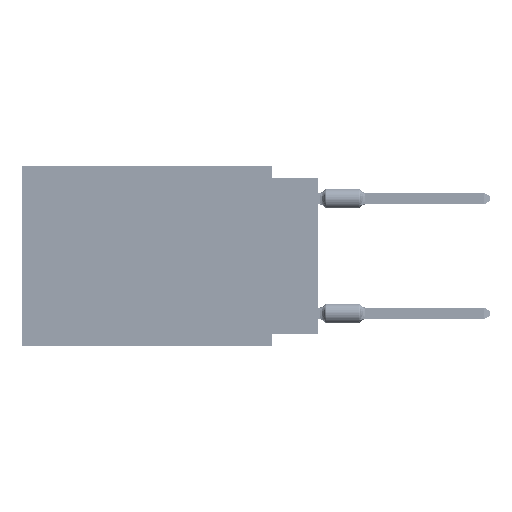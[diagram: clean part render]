
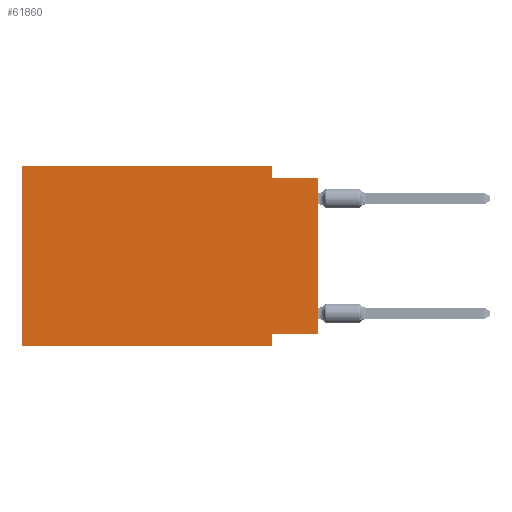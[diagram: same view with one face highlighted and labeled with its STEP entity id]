
A CAD part, left-side view. The second image highlights one B-rep face of the part: STEP entity #61860.
In plain terms, the highlighted planar face has unit normal (-1, 0, 0).
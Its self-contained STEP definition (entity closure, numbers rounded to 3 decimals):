
#1295 = VECTOR ( 'NONE', #41503, 1000. ) ;
#2583 = EDGE_CURVE ( 'NONE', #37512, #4246, #33294, .T. ) ;
#3146 = VERTEX_POINT ( 'NONE', #15341 ) ;
#3644 = ORIENTED_EDGE ( 'NONE', *, *, #2583, .T. ) ;
#4246 = VERTEX_POINT ( 'NONE', #16234 ) ;
#6691 = CARTESIAN_POINT ( 'NONE',  ( 0., 2.54, -0.635 ) ) ;
#6710 = LINE ( 'NONE', #60498, #7490 ) ;
#6810 = VERTEX_POINT ( 'NONE', #16343 ) ;
#7490 = VECTOR ( 'NONE', #61202, 1000. ) ;
#10549 = ORIENTED_EDGE ( 'NONE', *, *, #47215, .F. ) ;
#11896 = DIRECTION ( 'NONE',  ( 0., -1., 0. ) ) ;
#12000 = LINE ( 'NONE', #35159, #28196 ) ;
#12477 = EDGE_LOOP ( 'NONE', ( #29565, #55095, #37038, #61664, #54907, #3644, #34938, #10549 ) ) ;
#14765 = LINE ( 'NONE', #30801, #1295 ) ;
#14795 = VECTOR ( 'NONE', #61112, 1000. ) ;
#15341 = CARTESIAN_POINT ( 'NONE',  ( 0., 2.54, 0. ) ) ;
#16234 = CARTESIAN_POINT ( 'NONE',  ( 0., 2.54, -9.906 ) ) ;
#16343 = CARTESIAN_POINT ( 'NONE',  ( 0., 0., -9.271 ) ) ;
#18685 = CARTESIAN_POINT ( 'NONE',  ( 0., 0., 0. ) ) ;
#18696 = EDGE_CURVE ( 'NONE', #56143, #4246, #24344, .T. ) ;
#19536 = AXIS2_PLACEMENT_3D ( 'NONE', #52893, #68945, #63595 ) ;
#20134 = VECTOR ( 'NONE', #57823, 1000. ) ;
#22353 = DIRECTION ( 'NONE',  ( 0., -1., 0. ) ) ;
#24344 = LINE ( 'NONE', #57120, #20134 ) ;
#25487 = VECTOR ( 'NONE', #69147, 1000. ) ;
#25639 = VERTEX_POINT ( 'NONE', #51224 ) ;
#26032 = CARTESIAN_POINT ( 'NONE',  ( 0., 2.54, 0. ) ) ;
#26712 = EDGE_CURVE ( 'NONE', #37906, #68034, #6710, .T. ) ;
#28196 = VECTOR ( 'NONE', #45496, 1000. ) ;
#29565 = ORIENTED_EDGE ( 'NONE', *, *, #33624, .T. ) ;
#30801 = CARTESIAN_POINT ( 'NONE',  ( 0., 16.383, 0. ) ) ;
#33294 = LINE ( 'NONE', #60710, #57175 ) ;
#33624 = EDGE_CURVE ( 'NONE', #6810, #68034, #56103, .T. ) ;
#34938 = ORIENTED_EDGE ( 'NONE', *, *, #18696, .F. ) ;
#35159 = CARTESIAN_POINT ( 'NONE',  ( 0., 0., -9.271 ) ) ;
#35819 = PLANE ( 'NONE',  #19536 ) ;
#37038 = ORIENTED_EDGE ( 'NONE', *, *, #63046, .F. ) ;
#37512 = VERTEX_POINT ( 'NONE', #61271 ) ;
#37825 = EDGE_CURVE ( 'NONE', #25639, #3146, #43754, .T. ) ;
#37906 = VERTEX_POINT ( 'NONE', #6691 ) ;
#39091 = VECTOR ( 'NONE', #22353, 1000. ) ;
#41503 = DIRECTION ( 'NONE',  ( 0., 0., 1. ) ) ;
#42536 = CARTESIAN_POINT ( 'NONE',  ( 0., 0., -0.635 ) ) ;
#43754 = LINE ( 'NONE', #49436, #39091 ) ;
#45496 = DIRECTION ( 'NONE',  ( 0., 1., 0. ) ) ;
#47215 = EDGE_CURVE ( 'NONE', #6810, #56143, #12000, .T. ) ;
#49436 = CARTESIAN_POINT ( 'NONE',  ( 0., 16.383, 0. ) ) ;
#51224 = CARTESIAN_POINT ( 'NONE',  ( 0., 16.383, 0. ) ) ;
#51861 = EDGE_CURVE ( 'NONE', #37512, #25639, #14765, .T. ) ;
#52893 = CARTESIAN_POINT ( 'NONE',  ( 0., 16.383, 0. ) ) ;
#54907 = ORIENTED_EDGE ( 'NONE', *, *, #51861, .F. ) ;
#55095 = ORIENTED_EDGE ( 'NONE', *, *, #26712, .F. ) ;
#56103 = LINE ( 'NONE', #18685, #14795 ) ;
#56143 = VERTEX_POINT ( 'NONE', #62758 ) ;
#57120 = CARTESIAN_POINT ( 'NONE',  ( 0., 2.54, -9.906 ) ) ;
#57175 = VECTOR ( 'NONE', #11896, 1000. ) ;
#57193 = FACE_OUTER_BOUND ( 'NONE', #12477, .T. ) ;
#57823 = DIRECTION ( 'NONE',  ( 0., 0., -1. ) ) ;
#60498 = CARTESIAN_POINT ( 'NONE',  ( 0., 0., -0.635 ) ) ;
#60710 = CARTESIAN_POINT ( 'NONE',  ( 0., 16.383, -9.906 ) ) ;
#61112 = DIRECTION ( 'NONE',  ( 0., 0., 1. ) ) ;
#61202 = DIRECTION ( 'NONE',  ( 0., -1., 0. ) ) ;
#61271 = CARTESIAN_POINT ( 'NONE',  ( 0., 16.383, -9.906 ) ) ;
#61664 = ORIENTED_EDGE ( 'NONE', *, *, #37825, .F. ) ;
#61860 = ADVANCED_FACE ( 'NONE', ( #57193 ), #35819, .F. ) ;
#62758 = CARTESIAN_POINT ( 'NONE',  ( 0., 2.54, -9.271 ) ) ;
#63046 = EDGE_CURVE ( 'NONE', #3146, #37906, #68782, .T. ) ;
#63595 = DIRECTION ( 'NONE',  ( 0., 0., -1. ) ) ;
#68034 = VERTEX_POINT ( 'NONE', #42536 ) ;
#68782 = LINE ( 'NONE', #26032, #25487 ) ;
#68945 = DIRECTION ( 'NONE',  ( 1., 0., 0. ) ) ;
#69147 = DIRECTION ( 'NONE',  ( 0., 0., -1. ) ) ;
